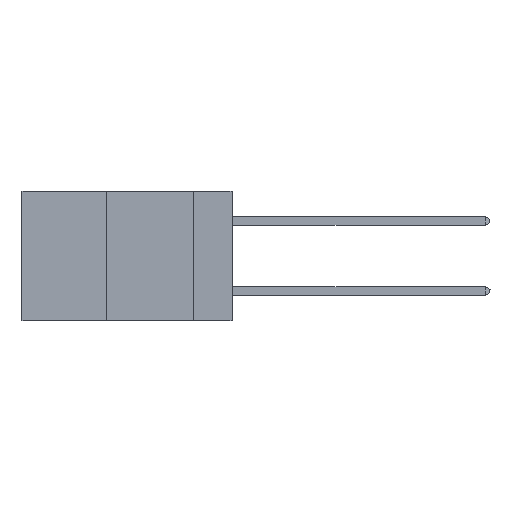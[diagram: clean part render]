
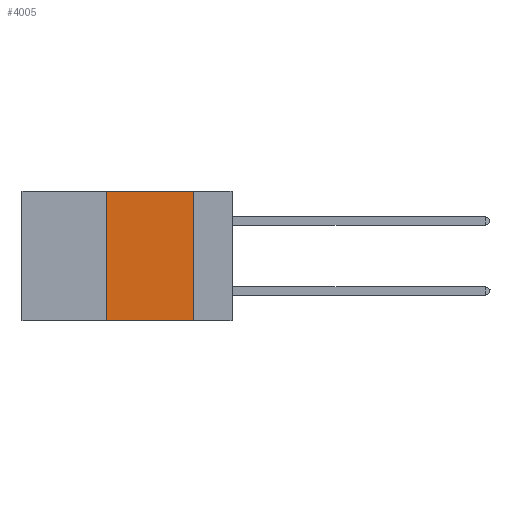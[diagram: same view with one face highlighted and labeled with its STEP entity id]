
A CAD part, left-side view. The second image highlights one B-rep face of the part: STEP entity #4005.
In plain terms, the highlighted planar face has unit normal (-1, 0, 0).
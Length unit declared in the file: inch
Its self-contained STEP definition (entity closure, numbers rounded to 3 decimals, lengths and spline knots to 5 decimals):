
#203 = VERTEX_POINT ( 'NONE', #17705 ) ;
#755 = VERTEX_POINT ( 'NONE', #18696 ) ;
#2876 = ORIENTED_EDGE ( 'NONE', *, *, #11590, .F. ) ;
#4005 = ADVANCED_FACE ( 'NONE', ( #21737 ), #19016, .F. ) ;
#4788 = ORIENTED_EDGE ( 'NONE', *, *, #19868, .F. ) ;
#5341 = ORIENTED_EDGE ( 'NONE', *, *, #21299, .F. ) ;
#6413 = DIRECTION ( 'NONE',  ( 0., -1., 0. ) ) ;
#8298 = LINE ( 'NONE', #24723, #25058 ) ;
#9615 = CARTESIAN_POINT ( 'NONE',  ( 0., 0.11, -0.37 ) ) ;
#10229 = AXIS2_PLACEMENT_3D ( 'NONE', #19183, #23255, #10672 ) ;
#10265 = CARTESIAN_POINT ( 'NONE',  ( 0., 0.6, -0.37 ) ) ;
#10672 = DIRECTION ( 'NONE',  ( 0., 0., -1. ) ) ;
#10828 = EDGE_CURVE ( 'NONE', #203, #26317, #20129, .T. ) ;
#11439 = LINE ( 'NONE', #14559, #12398 ) ;
#11590 = EDGE_CURVE ( 'NONE', #203, #755, #8298, .T. ) ;
#12277 = VECTOR ( 'NONE', #23025, 39.37008 ) ;
#12398 = VECTOR ( 'NONE', #6413, 39.37008 ) ;
#12628 = LINE ( 'NONE', #13836, #19506 ) ;
#13836 = CARTESIAN_POINT ( 'NONE',  ( 0., 0.11, 0. ) ) ;
#14208 = DIRECTION ( 'NONE',  ( 0., 0., 1. ) ) ;
#14559 = CARTESIAN_POINT ( 'NONE',  ( 0., 0.6, 0. ) ) ;
#17630 = DIRECTION ( 'NONE',  ( 0., 0., -1. ) ) ;
#17705 = CARTESIAN_POINT ( 'NONE',  ( 0., 0.36, -0.37 ) ) ;
#18696 = CARTESIAN_POINT ( 'NONE',  ( 0., 0.36, 0. ) ) ;
#18868 = ORIENTED_EDGE ( 'NONE', *, *, #10828, .T. ) ;
#19010 = VERTEX_POINT ( 'NONE', #22090 ) ;
#19016 = PLANE ( 'NONE',  #10229 ) ;
#19183 = CARTESIAN_POINT ( 'NONE',  ( 0., 0.6, 0. ) ) ;
#19506 = VECTOR ( 'NONE', #17630, 39.37008 ) ;
#19868 = EDGE_CURVE ( 'NONE', #755, #19010, #11439, .T. ) ;
#20129 = LINE ( 'NONE', #10265, #12277 ) ;
#21299 = EDGE_CURVE ( 'NONE', #19010, #26317, #12628, .T. ) ;
#21737 = FACE_OUTER_BOUND ( 'NONE', #26803, .T. ) ;
#22090 = CARTESIAN_POINT ( 'NONE',  ( 0., 0.11, 0. ) ) ;
#23025 = DIRECTION ( 'NONE',  ( 0., -1., 0. ) ) ;
#23255 = DIRECTION ( 'NONE',  ( 1., 0., 0. ) ) ;
#24723 = CARTESIAN_POINT ( 'NONE',  ( 0., 0.36, 0. ) ) ;
#25058 = VECTOR ( 'NONE', #14208, 39.37008 ) ;
#26317 = VERTEX_POINT ( 'NONE', #9615 ) ;
#26803 = EDGE_LOOP ( 'NONE', ( #5341, #4788, #2876, #18868 ) ) ;
